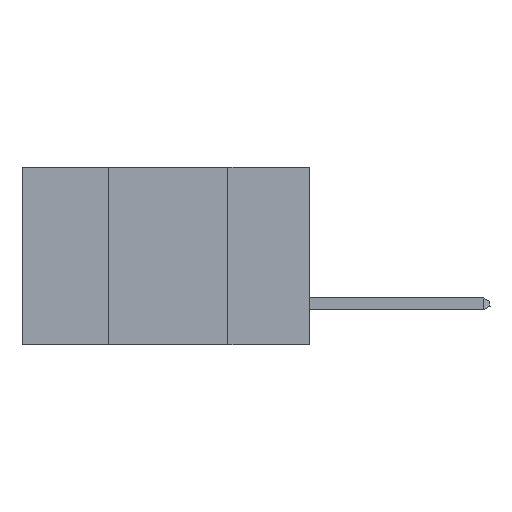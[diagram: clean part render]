
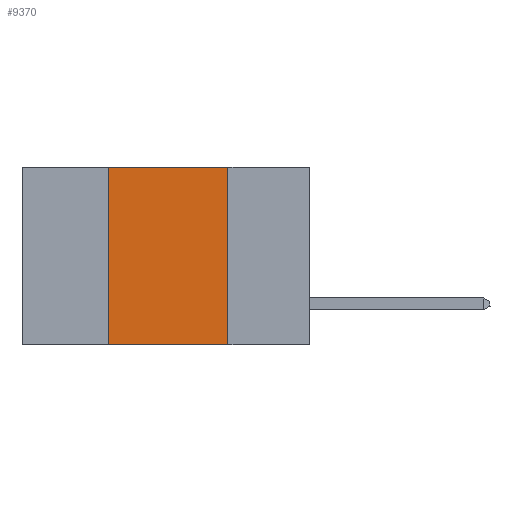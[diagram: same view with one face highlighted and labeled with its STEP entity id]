
A CAD part, left-side view. The second image highlights one B-rep face of the part: STEP entity #9370.
In plain terms, the highlighted planar face has unit normal (-1, 0, 0).
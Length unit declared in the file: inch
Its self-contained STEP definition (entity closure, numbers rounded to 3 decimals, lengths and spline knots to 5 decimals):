
#619 = VECTOR ( 'NONE', #7927, 39.37008 ) ;
#635 = CARTESIAN_POINT ( 'NONE',  ( 0., 0.42, 0. ) ) ;
#776 = ORIENTED_EDGE ( 'NONE', *, *, #3024, .F. ) ;
#779 = AXIS2_PLACEMENT_3D ( 'NONE', #6590, #9471, #4735 ) ;
#870 = ORIENTED_EDGE ( 'NONE', *, *, #3539, .F. ) ;
#1322 = VERTEX_POINT ( 'NONE', #635 ) ;
#1671 = PLANE ( 'NONE',  #779 ) ;
#2577 = CARTESIAN_POINT ( 'NONE',  ( 0., 0.6, -0.37 ) ) ;
#2702 = VERTEX_POINT ( 'NONE', #5505 ) ;
#3024 = EDGE_CURVE ( 'NONE', #3424, #1322, #7906, .T. ) ;
#3078 = VECTOR ( 'NONE', #9363, 39.37008 ) ;
#3171 = CARTESIAN_POINT ( 'NONE',  ( 0., 0.42, 0. ) ) ;
#3424 = VERTEX_POINT ( 'NONE', #6984 ) ;
#3539 = EDGE_CURVE ( 'NONE', #1322, #9941, #9759, .T. ) ;
#3650 = ORIENTED_EDGE ( 'NONE', *, *, #6663, .F. ) ;
#3889 = EDGE_CURVE ( 'NONE', #3424, #2702, #5698, .T. ) ;
#3930 = FACE_OUTER_BOUND ( 'NONE', #6366, .T. ) ;
#4735 = DIRECTION ( 'NONE',  ( 0., 0., -1. ) ) ;
#5505 = CARTESIAN_POINT ( 'NONE',  ( 0., 0.17, -0.37 ) ) ;
#5698 = LINE ( 'NONE', #2577, #619 ) ;
#5781 = CARTESIAN_POINT ( 'NONE',  ( 0., 0.6, 0. ) ) ;
#6163 = LINE ( 'NONE', #6861, #7147 ) ;
#6366 = EDGE_LOOP ( 'NONE', ( #3650, #870, #776, #6792 ) ) ;
#6590 = CARTESIAN_POINT ( 'NONE',  ( 0., 0.6, 0. ) ) ;
#6663 = EDGE_CURVE ( 'NONE', #9941, #2702, #6163, .T. ) ;
#6792 = ORIENTED_EDGE ( 'NONE', *, *, #3889, .T. ) ;
#6861 = CARTESIAN_POINT ( 'NONE',  ( 0., 0.17, 0. ) ) ;
#6984 = CARTESIAN_POINT ( 'NONE',  ( 0., 0.42, -0.37 ) ) ;
#7147 = VECTOR ( 'NONE', #8427, 39.37008 ) ;
#7906 = LINE ( 'NONE', #3171, #3078 ) ;
#7927 = DIRECTION ( 'NONE',  ( 0., -1., 0. ) ) ;
#7929 = VECTOR ( 'NONE', #9707, 39.37008 ) ;
#8332 = CARTESIAN_POINT ( 'NONE',  ( 0., 0.17, 0. ) ) ;
#8427 = DIRECTION ( 'NONE',  ( 0., 0., -1. ) ) ;
#9363 = DIRECTION ( 'NONE',  ( 0., 0., 1. ) ) ;
#9370 = ADVANCED_FACE ( 'NONE', ( #3930 ), #1671, .F. ) ;
#9471 = DIRECTION ( 'NONE',  ( 1., 0., 0. ) ) ;
#9707 = DIRECTION ( 'NONE',  ( 0., -1., 0. ) ) ;
#9759 = LINE ( 'NONE', #5781, #7929 ) ;
#9941 = VERTEX_POINT ( 'NONE', #8332 ) ;
